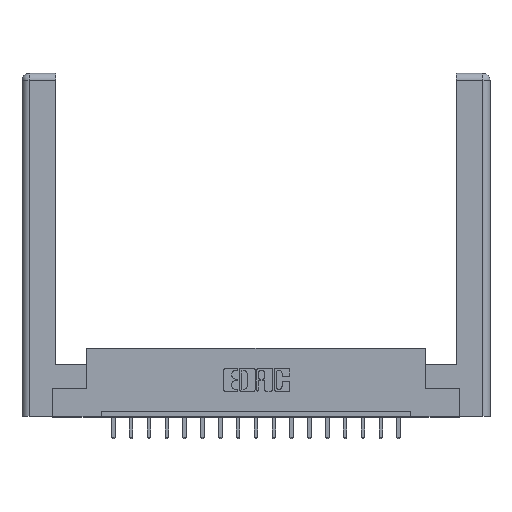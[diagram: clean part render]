
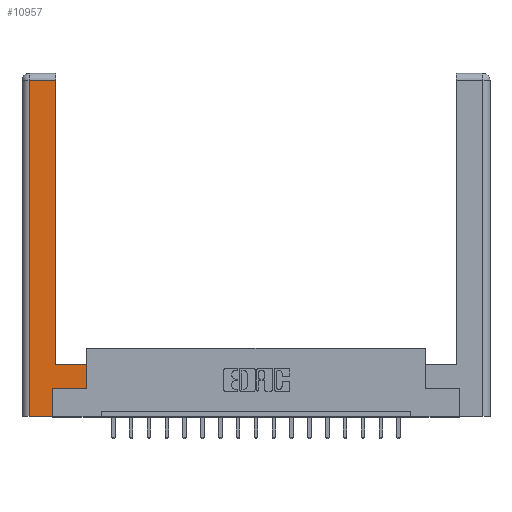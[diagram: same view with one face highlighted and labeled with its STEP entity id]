
A CAD part, top view. The second image highlights one B-rep face of the part: STEP entity #10957.
In plain terms, the highlighted planar face has unit normal (0, 0, 1).
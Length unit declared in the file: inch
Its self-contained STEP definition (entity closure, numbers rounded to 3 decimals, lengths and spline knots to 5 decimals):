
#97 = LINE ( 'NONE', #10344, #2340 ) ;
#472 = CARTESIAN_POINT ( 'NONE',  ( 0.265, 0., 0. ) ) ;
#561 = VERTEX_POINT ( 'NONE', #10884 ) ;
#572 = VERTEX_POINT ( 'NONE', #15306 ) ;
#966 = CARTESIAN_POINT ( 'NONE',  ( 0.0615, 0., 0. ) ) ;
#1384 = DIRECTION ( 'NONE',  ( -1., 0., 0. ) ) ;
#1439 = CARTESIAN_POINT ( 'NONE',  ( 0.295, 3., 0. ) ) ;
#1485 = ORIENTED_EDGE ( 'NONE', *, *, #15507, .T. ) ;
#1599 = DIRECTION ( 'NONE',  ( 0., 1., 0. ) ) ;
#1863 = VERTEX_POINT ( 'NONE', #17912 ) ;
#1870 = PLANE ( 'NONE',  #6727 ) ;
#1918 = DIRECTION ( 'NONE',  ( 1., 0., 0. ) ) ;
#2294 = EDGE_CURVE ( 'NONE', #572, #9611, #6279, .T. ) ;
#2340 = VECTOR ( 'NONE', #6112, 39.37008 ) ;
#2376 = EDGE_CURVE ( 'NONE', #5331, #3722, #5841, .T. ) ;
#2690 = LINE ( 'NONE', #9961, #9417 ) ;
#2777 = DIRECTION ( 'NONE',  ( 0., 1., 0. ) ) ;
#3565 = ORIENTED_EDGE ( 'NONE', *, *, #6041, .T. ) ;
#3722 = VERTEX_POINT ( 'NONE', #10973 ) ;
#3853 = CARTESIAN_POINT ( 'NONE',  ( 0.0615, 0., 0. ) ) ;
#3946 = VECTOR ( 'NONE', #5967, 39.37008 ) ;
#4476 = EDGE_CURVE ( 'NONE', #9611, #5331, #7358, .T. ) ;
#5002 = CARTESIAN_POINT ( 'NONE',  ( 0.295, 0.45, 0. ) ) ;
#5331 = VERTEX_POINT ( 'NONE', #966 ) ;
#5841 = LINE ( 'NONE', #472, #16191 ) ;
#5967 = DIRECTION ( 'NONE',  ( 1., 0., 0. ) ) ;
#6041 = EDGE_CURVE ( 'NONE', #10128, #10385, #97, .T. ) ;
#6112 = DIRECTION ( 'NONE',  ( -1., 0., 0. ) ) ;
#6116 = ORIENTED_EDGE ( 'NONE', *, *, #2376, .T. ) ;
#6279 = LINE ( 'NONE', #17161, #12588 ) ;
#6654 = LINE ( 'NONE', #15547, #3946 ) ;
#6680 = EDGE_LOOP ( 'NONE', ( #13775, #7850, #14475, #6116, #12603, #16085, #1485, #3565 ) ) ;
#6727 = AXIS2_PLACEMENT_3D ( 'NONE', #18160, #10784, #12371 ) ;
#7358 = LINE ( 'NONE', #3853, #15663 ) ;
#7850 = ORIENTED_EDGE ( 'NONE', *, *, #2294, .T. ) ;
#7878 = LINE ( 'NONE', #1439, #18006 ) ;
#8173 = DIRECTION ( 'NONE',  ( 0., -1., 0. ) ) ;
#8328 = EDGE_CURVE ( 'NONE', #1863, #561, #6654, .T. ) ;
#8561 = VECTOR ( 'NONE', #14588, 39.37008 ) ;
#8689 = CARTESIAN_POINT ( 'NONE',  ( 0.0615, 2.94, 0. ) ) ;
#9246 = FACE_OUTER_BOUND ( 'NONE', #6680, .T. ) ;
#9417 = VECTOR ( 'NONE', #1599, 39.37008 ) ;
#9611 = VERTEX_POINT ( 'NONE', #8689 ) ;
#9961 = CARTESIAN_POINT ( 'NONE',  ( 0.265, 0.245, 0. ) ) ;
#10128 = VERTEX_POINT ( 'NONE', #12332 ) ;
#10134 = LINE ( 'NONE', #12955, #8561 ) ;
#10344 = CARTESIAN_POINT ( 'NONE',  ( 0.295, 0.45, 0. ) ) ;
#10385 = VERTEX_POINT ( 'NONE', #5002 ) ;
#10784 = DIRECTION ( 'NONE',  ( 0., 0., -1. ) ) ;
#10884 = CARTESIAN_POINT ( 'NONE',  ( 0.565, 0.245, 0. ) ) ;
#10957 = ADVANCED_FACE ( 'NONE', ( #9246 ), #1870, .F. ) ;
#10973 = CARTESIAN_POINT ( 'NONE',  ( 0.265, 0., 0. ) ) ;
#12303 = EDGE_CURVE ( 'NONE', #3722, #1863, #2690, .T. ) ;
#12332 = CARTESIAN_POINT ( 'NONE',  ( 0.565, 0.45, 0. ) ) ;
#12371 = DIRECTION ( 'NONE',  ( -1., 0., 0. ) ) ;
#12588 = VECTOR ( 'NONE', #1384, 39.37008 ) ;
#12603 = ORIENTED_EDGE ( 'NONE', *, *, #12303, .T. ) ;
#12955 = CARTESIAN_POINT ( 'NONE',  ( 0.565, 0.45, 0. ) ) ;
#13775 = ORIENTED_EDGE ( 'NONE', *, *, #15405, .T. ) ;
#14475 = ORIENTED_EDGE ( 'NONE', *, *, #4476, .T. ) ;
#14588 = DIRECTION ( 'NONE',  ( 0., 1., 0. ) ) ;
#15306 = CARTESIAN_POINT ( 'NONE',  ( 0.295, 2.94, 0. ) ) ;
#15405 = EDGE_CURVE ( 'NONE', #10385, #572, #7878, .T. ) ;
#15507 = EDGE_CURVE ( 'NONE', #561, #10128, #10134, .T. ) ;
#15547 = CARTESIAN_POINT ( 'NONE',  ( 0.565, 0.245, 0. ) ) ;
#15663 = VECTOR ( 'NONE', #8173, 39.37008 ) ;
#16085 = ORIENTED_EDGE ( 'NONE', *, *, #8328, .T. ) ;
#16191 = VECTOR ( 'NONE', #1918, 39.37008 ) ;
#17161 = CARTESIAN_POINT ( 'NONE',  ( 0.0615, 2.94, 0. ) ) ;
#17912 = CARTESIAN_POINT ( 'NONE',  ( 0.265, 0.245, 0. ) ) ;
#18006 = VECTOR ( 'NONE', #2777, 39.37008 ) ;
#18160 = CARTESIAN_POINT ( 'NONE',  ( 0., 0., 0. ) ) ;
